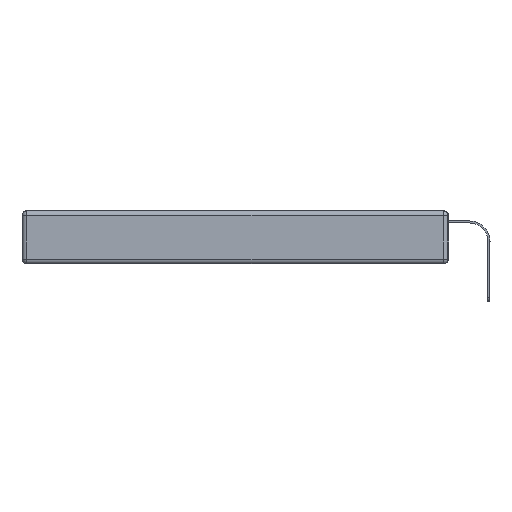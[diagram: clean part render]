
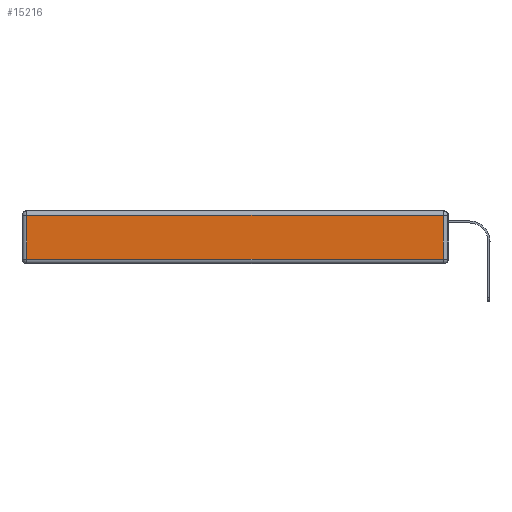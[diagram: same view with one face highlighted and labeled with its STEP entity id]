
A CAD part, left-side view. The second image highlights one B-rep face of the part: STEP entity #15216.
In plain terms, the highlighted planar face has unit normal (-1, 0, 0).
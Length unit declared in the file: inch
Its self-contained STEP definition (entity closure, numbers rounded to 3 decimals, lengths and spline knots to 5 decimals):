
#290 = ORIENTED_EDGE ( 'NONE', *, *, #16485, .T. ) ;
#1053 = LINE ( 'NONE', #16077, #13774 ) ;
#1346 = CARTESIAN_POINT ( 'NONE',  ( 0., 0.03, -0.03 ) ) ;
#1489 = EDGE_CURVE ( 'NONE', #23555, #6775, #16134, .T. ) ;
#2101 = ORIENTED_EDGE ( 'NONE', *, *, #1489, .T. ) ;
#3671 = VECTOR ( 'NONE', #23132, 39.37008 ) ;
#4375 = CARTESIAN_POINT ( 'NONE',  ( 0., 2.75, -0.03 ) ) ;
#5083 = DIRECTION ( 'NONE',  ( 0., -1., 0. ) ) ;
#6362 = CARTESIAN_POINT ( 'NONE',  ( 0., 2.72, -0.03 ) ) ;
#6775 = VERTEX_POINT ( 'NONE', #6362 ) ;
#8081 = VERTEX_POINT ( 'NONE', #14959 ) ;
#8738 = DIRECTION ( 'NONE',  ( 0., 0., 1. ) ) ;
#8748 = LINE ( 'NONE', #14694, #20605 ) ;
#9875 = DIRECTION ( 'NONE',  ( -1., 0., 0. ) ) ;
#11748 = FACE_OUTER_BOUND ( 'NONE', #18761, .T. ) ;
#12026 = VECTOR ( 'NONE', #12458, 39.37008 ) ;
#12117 = PLANE ( 'NONE',  #19387 ) ;
#12226 = ORIENTED_EDGE ( 'NONE', *, *, #16725, .T. ) ;
#12458 = DIRECTION ( 'NONE',  ( 0., 1., 0. ) ) ;
#13645 = CARTESIAN_POINT ( 'NONE',  ( 0., 0., -0.343 ) ) ;
#13689 = CARTESIAN_POINT ( 'NONE',  ( 0., 2.72, -0.313 ) ) ;
#13774 = VECTOR ( 'NONE', #8738, 39.37008 ) ;
#14694 = CARTESIAN_POINT ( 'NONE',  ( 0., 0., -0.313 ) ) ;
#14959 = CARTESIAN_POINT ( 'NONE',  ( 0., 0.03, -0.313 ) ) ;
#15216 = ADVANCED_FACE ( 'NONE', ( #11748 ), #12117, .T. ) ;
#15434 = CARTESIAN_POINT ( 'NONE',  ( 0., 2.72, -0.343 ) ) ;
#16077 = CARTESIAN_POINT ( 'NONE',  ( 0., 0.03, -0.343 ) ) ;
#16134 = LINE ( 'NONE', #4375, #12026 ) ;
#16485 = EDGE_CURVE ( 'NONE', #8081, #23555, #1053, .T. ) ;
#16725 = EDGE_CURVE ( 'NONE', #6775, #23860, #21830, .T. ) ;
#18761 = EDGE_LOOP ( 'NONE', ( #20736, #290, #2101, #12226 ) ) ;
#19387 = AXIS2_PLACEMENT_3D ( 'NONE', #13645, #9875, #23250 ) ;
#20605 = VECTOR ( 'NONE', #5083, 39.37008 ) ;
#20736 = ORIENTED_EDGE ( 'NONE', *, *, #21932, .T. ) ;
#21830 = LINE ( 'NONE', #15434, #3671 ) ;
#21932 = EDGE_CURVE ( 'NONE', #23860, #8081, #8748, .T. ) ;
#23132 = DIRECTION ( 'NONE',  ( 0., 0., -1. ) ) ;
#23250 = DIRECTION ( 'NONE',  ( 0., 0., 1. ) ) ;
#23555 = VERTEX_POINT ( 'NONE', #1346 ) ;
#23860 = VERTEX_POINT ( 'NONE', #13689 ) ;
